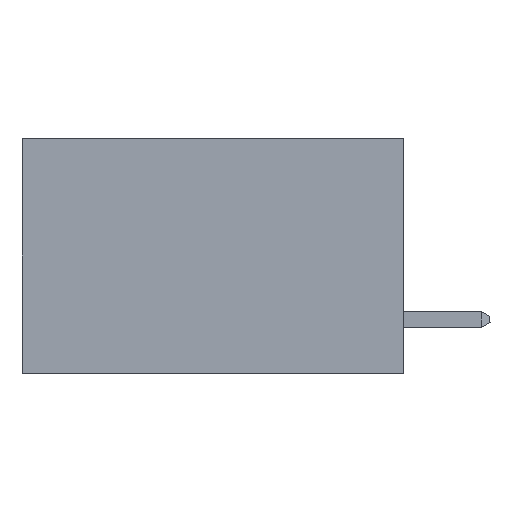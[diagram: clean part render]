
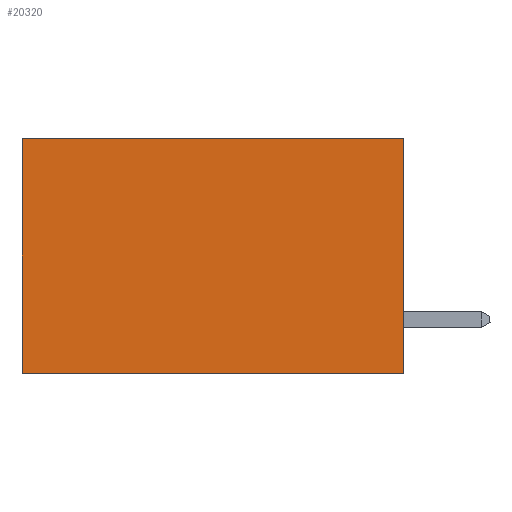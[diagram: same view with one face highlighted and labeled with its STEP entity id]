
A CAD part, left-side view. The second image highlights one B-rep face of the part: STEP entity #20320.
In plain terms, the highlighted planar face has unit normal (-1, 0, 0).
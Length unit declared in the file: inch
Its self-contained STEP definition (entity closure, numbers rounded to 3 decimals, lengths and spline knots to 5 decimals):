
#378 = PLANE ( 'NONE',  #5956 ) ;
#520 = CARTESIAN_POINT ( 'NONE',  ( 0.2875, 0.6, -0.37 ) ) ;
#1474 = DIRECTION ( 'NONE',  ( 0., 1., 0. ) ) ;
#1565 = LINE ( 'NONE', #2958, #17666 ) ;
#1595 = EDGE_CURVE ( 'NONE', #3602, #15904, #1762, .T. ) ;
#1634 = CARTESIAN_POINT ( 'NONE',  ( 0.2875, 0., 0. ) ) ;
#1762 = LINE ( 'NONE', #12948, #3288 ) ;
#1969 = DIRECTION ( 'NONE',  ( 0., 0., -1. ) ) ;
#2092 = CARTESIAN_POINT ( 'NONE',  ( 0.2875, 0.6, 0. ) ) ;
#2488 = FACE_OUTER_BOUND ( 'NONE', #6072, .T. ) ;
#2958 = CARTESIAN_POINT ( 'NONE',  ( 0.2875, 0.6, 0. ) ) ;
#3112 = DIRECTION ( 'NONE',  ( 0., 0., -1. ) ) ;
#3288 = VECTOR ( 'NONE', #1474, 39.37008 ) ;
#3469 = LINE ( 'NONE', #1634, #7026 ) ;
#3602 = VERTEX_POINT ( 'NONE', #5825 ) ;
#5321 = CARTESIAN_POINT ( 'NONE',  ( 0.2875, 0., 0. ) ) ;
#5601 = ORIENTED_EDGE ( 'NONE', *, *, #8173, .T. ) ;
#5825 = CARTESIAN_POINT ( 'NONE',  ( 0.2875, 0., -0.37 ) ) ;
#5956 = AXIS2_PLACEMENT_3D ( 'NONE', #5321, #16544, #6739 ) ;
#6072 = EDGE_LOOP ( 'NONE', ( #17654, #16764, #9540, #5601 ) ) ;
#6739 = DIRECTION ( 'NONE',  ( 0., 0., -1. ) ) ;
#7026 = VECTOR ( 'NONE', #1969, 39.37008 ) ;
#8173 = EDGE_CURVE ( 'NONE', #14915, #8299, #9136, .T. ) ;
#8299 = VERTEX_POINT ( 'NONE', #2092 ) ;
#8940 = EDGE_CURVE ( 'NONE', #8299, #15904, #1565, .T. ) ;
#9136 = LINE ( 'NONE', #14542, #19426 ) ;
#9540 = ORIENTED_EDGE ( 'NONE', *, *, #10791, .F. ) ;
#9580 = DIRECTION ( 'NONE',  ( 0., 1., 0. ) ) ;
#10791 = EDGE_CURVE ( 'NONE', #14915, #3602, #3469, .T. ) ;
#12948 = CARTESIAN_POINT ( 'NONE',  ( 0.2875, 0., -0.37 ) ) ;
#14542 = CARTESIAN_POINT ( 'NONE',  ( 0.2875, 0., 0. ) ) ;
#14915 = VERTEX_POINT ( 'NONE', #18287 ) ;
#15904 = VERTEX_POINT ( 'NONE', #520 ) ;
#16544 = DIRECTION ( 'NONE',  ( 1., 0., 0. ) ) ;
#16764 = ORIENTED_EDGE ( 'NONE', *, *, #1595, .F. ) ;
#17654 = ORIENTED_EDGE ( 'NONE', *, *, #8940, .T. ) ;
#17666 = VECTOR ( 'NONE', #3112, 39.37008 ) ;
#18287 = CARTESIAN_POINT ( 'NONE',  ( 0.2875, 0., 0. ) ) ;
#19426 = VECTOR ( 'NONE', #9580, 39.37008 ) ;
#20320 = ADVANCED_FACE ( 'NONE', ( #2488 ), #378, .F. ) ;
